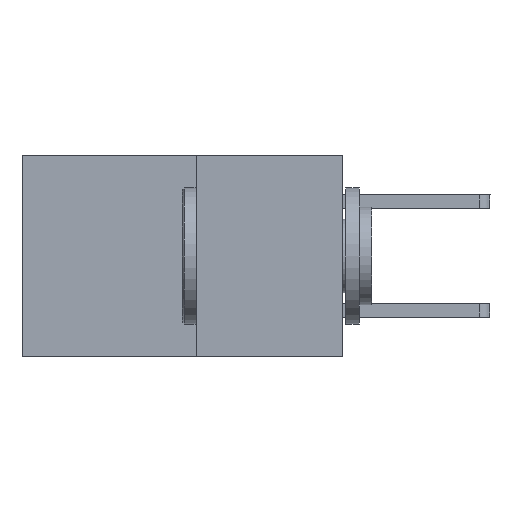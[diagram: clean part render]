
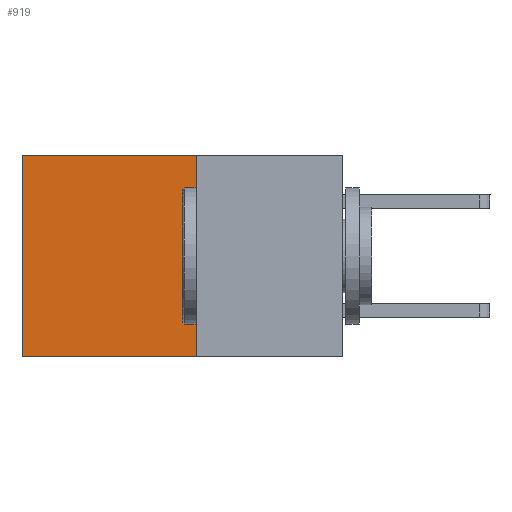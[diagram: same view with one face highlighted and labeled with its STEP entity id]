
A CAD part, left-side view. The second image highlights one B-rep face of the part: STEP entity #919.
In plain terms, the highlighted planar face has unit normal (-1, 0, 0).
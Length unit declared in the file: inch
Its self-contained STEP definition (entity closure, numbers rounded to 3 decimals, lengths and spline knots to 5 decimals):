
#218 = LINE ( 'NONE', #3768, #7559 ) ;
#259 = VERTEX_POINT ( 'NONE', #4913 ) ;
#279 = ORIENTED_EDGE ( 'NONE', *, *, #7286, .F. ) ;
#324 = VECTOR ( 'NONE', #4607, 39.37008 ) ;
#689 = CARTESIAN_POINT ( 'NONE',  ( 0.277, 0.27, -0.37 ) ) ;
#894 = DIRECTION ( 'NONE',  ( 0., 0., -1. ) ) ;
#895 = EDGE_LOOP ( 'NONE', ( #2094, #4032, #279, #7340 ) ) ;
#919 = ADVANCED_FACE ( 'NONE', ( #9135 ), #1966, .F. ) ;
#1028 = VECTOR ( 'NONE', #9264, 39.37008 ) ;
#1681 = LINE ( 'NONE', #4704, #324 ) ;
#1966 = PLANE ( 'NONE',  #6752 ) ;
#2094 = ORIENTED_EDGE ( 'NONE', *, *, #3794, .T. ) ;
#2521 = EDGE_CURVE ( 'NONE', #8418, #5471, #1681, .T. ) ;
#3352 = CARTESIAN_POINT ( 'NONE',  ( 0.277, 0.59, -0.37 ) ) ;
#3609 = DIRECTION ( 'NONE',  ( 0., 1., 0. ) ) ;
#3768 = CARTESIAN_POINT ( 'NONE',  ( 0.277, 0.27, -0.37 ) ) ;
#3794 = EDGE_CURVE ( 'NONE', #5471, #8583, #4072, .T. ) ;
#3979 = CARTESIAN_POINT ( 'NONE',  ( 0.277, 0.59, -0.37 ) ) ;
#4032 = ORIENTED_EDGE ( 'NONE', *, *, #5919, .F. ) ;
#4072 = LINE ( 'NONE', #3979, #1028 ) ;
#4082 = DIRECTION ( 'NONE',  ( 0., 0., -1. ) ) ;
#4607 = DIRECTION ( 'NONE',  ( 0., 1., 0. ) ) ;
#4652 = CARTESIAN_POINT ( 'NONE',  ( 0.277, 0.59, 0. ) ) ;
#4704 = CARTESIAN_POINT ( 'NONE',  ( 0.277, 0.27, 0. ) ) ;
#4913 = CARTESIAN_POINT ( 'NONE',  ( 0.277, 0.27, -0.37 ) ) ;
#5471 = VERTEX_POINT ( 'NONE', #4652 ) ;
#5673 = DIRECTION ( 'NONE',  ( 1., 0., 0. ) ) ;
#5919 = EDGE_CURVE ( 'NONE', #259, #8583, #8667, .T. ) ;
#6205 = CARTESIAN_POINT ( 'NONE',  ( 0.277, 0.27, -0.37 ) ) ;
#6739 = VECTOR ( 'NONE', #3609, 39.37008 ) ;
#6752 = AXIS2_PLACEMENT_3D ( 'NONE', #6205, #5673, #4082 ) ;
#6879 = CARTESIAN_POINT ( 'NONE',  ( 0.277, 0.27, 0. ) ) ;
#7286 = EDGE_CURVE ( 'NONE', #8418, #259, #218, .T. ) ;
#7340 = ORIENTED_EDGE ( 'NONE', *, *, #2521, .T. ) ;
#7559 = VECTOR ( 'NONE', #894, 39.37008 ) ;
#8418 = VERTEX_POINT ( 'NONE', #6879 ) ;
#8583 = VERTEX_POINT ( 'NONE', #3352 ) ;
#8667 = LINE ( 'NONE', #689, #6739 ) ;
#9135 = FACE_OUTER_BOUND ( 'NONE', #895, .T. ) ;
#9264 = DIRECTION ( 'NONE',  ( 0., 0., -1. ) ) ;
